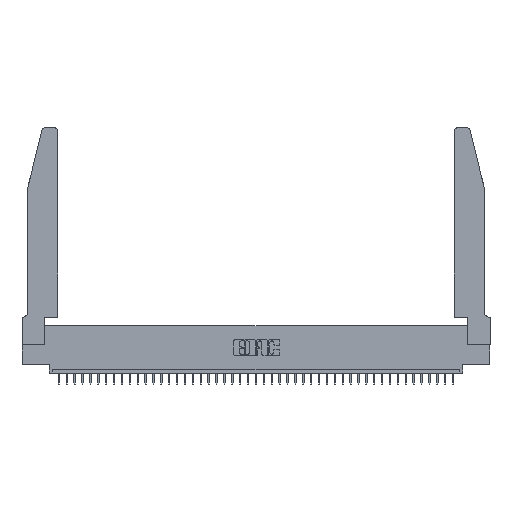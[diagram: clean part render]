
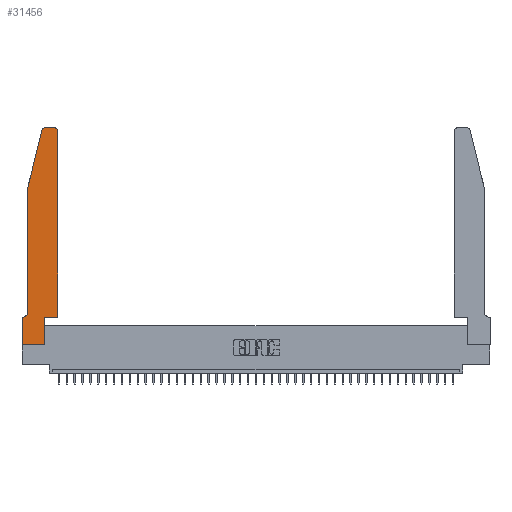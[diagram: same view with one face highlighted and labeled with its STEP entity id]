
A CAD part, top view. The second image highlights one B-rep face of the part: STEP entity #31456.
In plain terms, the highlighted planar face has unit normal (0, 0, 1).
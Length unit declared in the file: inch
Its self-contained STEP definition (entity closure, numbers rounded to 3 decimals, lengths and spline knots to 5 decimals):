
#606 = ORIENTED_EDGE ( 'NONE', *, *, #36842, .T. ) ;
#1045 = LINE ( 'NONE', #23851, #20287 ) ;
#1211 = ORIENTED_EDGE ( 'NONE', *, *, #30237, .T. ) ;
#1244 = CARTESIAN_POINT ( 'NONE',  ( 0.4505, 2.72, 0.37 ) ) ;
#2328 = LINE ( 'NONE', #15305, #37994 ) ;
#2401 = DIRECTION ( 'NONE',  ( 1., 0., 0. ) ) ;
#3042 = CARTESIAN_POINT ( 'NONE',  ( 0.0755, 2., 0.37 ) ) ;
#3442 = VERTEX_POINT ( 'NONE', #22814 ) ;
#3602 = VERTEX_POINT ( 'NONE', #1244 ) ;
#4045 = ORIENTED_EDGE ( 'NONE', *, *, #16039, .T. ) ;
#4070 = VECTOR ( 'NONE', #5723, 39.37008 ) ;
#4198 = ORIENTED_EDGE ( 'NONE', *, *, #23228, .T. ) ;
#4485 = VERTEX_POINT ( 'NONE', #30948 ) ;
#4670 = PLANE ( 'NONE',  #37816 ) ;
#5023 = ORIENTED_EDGE ( 'NONE', *, *, #5055, .T. ) ;
#5055 = EDGE_CURVE ( 'NONE', #14122, #22000, #2328, .T. ) ;
#5507 = EDGE_CURVE ( 'NONE', #41959, #19630, #41713, .T. ) ;
#5723 = DIRECTION ( 'NONE',  ( -1., 0., 0. ) ) ;
#5950 = EDGE_CURVE ( 'NONE', #22000, #36508, #8387, .T. ) ;
#6089 = CARTESIAN_POINT ( 'NONE',  ( 0.0755, 0.42, 0.37 ) ) ;
#6306 = CARTESIAN_POINT ( 'NONE',  ( 0.4205, 2.75, 0.37 ) ) ;
#6488 = EDGE_CURVE ( 'NONE', #36508, #39831, #25980, .T. ) ;
#6580 = DIRECTION ( 'NONE',  ( 1., 0., 0. ) ) ;
#6713 = VERTEX_POINT ( 'NONE', #30853 ) ;
#7894 = CARTESIAN_POINT ( 'NONE',  ( 0.4505, 0.35, 0.37 ) ) ;
#8236 = CARTESIAN_POINT ( 'NONE',  ( 0.0755, 0.35, 0.37 ) ) ;
#8387 = LINE ( 'NONE', #15000, #8738 ) ;
#8738 = VECTOR ( 'NONE', #38462, 39.37008 ) ;
#9120 = DIRECTION ( 'NONE',  ( 1., 0., 0. ) ) ;
#9305 = ORIENTED_EDGE ( 'NONE', *, *, #5507, .T. ) ;
#10061 = CARTESIAN_POINT ( 'NONE',  ( 0.0055, 0.42, 0.37 ) ) ;
#10127 = ORIENTED_EDGE ( 'NONE', *, *, #6488, .T. ) ;
#12064 = CARTESIAN_POINT ( 'NONE',  ( 0.2865, 0., 0.37 ) ) ;
#12339 = ORIENTED_EDGE ( 'NONE', *, *, #30399, .T. ) ;
#12459 = DIRECTION ( 'NONE',  ( 0., -1., 0. ) ) ;
#13036 = EDGE_CURVE ( 'NONE', #6713, #21126, #40873, .T. ) ;
#13082 = CARTESIAN_POINT ( 'NONE',  ( 0.0755, 2., 0.37 ) ) ;
#13480 = ORIENTED_EDGE ( 'NONE', *, *, #25115, .T. ) ;
#14122 = VERTEX_POINT ( 'NONE', #41504 ) ;
#15000 = CARTESIAN_POINT ( 'NONE',  ( 0.2865, 0.35, 0.37 ) ) ;
#15305 = CARTESIAN_POINT ( 'NONE',  ( 0., 0., 0.37 ) ) ;
#16039 = EDGE_CURVE ( 'NONE', #39831, #3602, #30928, .T. ) ;
#17051 = DIRECTION ( 'NONE',  ( 0., -1., 0. ) ) ;
#17083 = DIRECTION ( 'NONE',  ( -1., 0., 0. ) ) ;
#17135 = AXIS2_PLACEMENT_3D ( 'NONE', #31390, #18594, #2401 ) ;
#18223 = CARTESIAN_POINT ( 'NONE',  ( 0., 0.35, 0.37 ) ) ;
#18594 = DIRECTION ( 'NONE',  ( 0., 0., 1. ) ) ;
#18669 = DIRECTION ( 'NONE',  ( 1., 0., 0. ) ) ;
#19284 = VECTOR ( 'NONE', #28273, 39.37008 ) ;
#19527 = DIRECTION ( 'NONE',  ( 0., 0., 1. ) ) ;
#19536 = DIRECTION ( 'NONE',  ( 1., 0., 0. ) ) ;
#19630 = VERTEX_POINT ( 'NONE', #6089 ) ;
#19862 = CARTESIAN_POINT ( 'NONE',  ( 0.2865, 0.35, 0.37 ) ) ;
#20282 = DIRECTION ( 'NONE',  ( 0., 0., -1. ) ) ;
#20287 = VECTOR ( 'NONE', #17051, 39.37008 ) ;
#20351 = VECTOR ( 'NONE', #6580, 39.37008 ) ;
#20689 = CIRCLE ( 'NONE', #39810, 0.07 ) ;
#21126 = VERTEX_POINT ( 'NONE', #18223 ) ;
#22000 = VERTEX_POINT ( 'NONE', #12064 ) ;
#22293 = DIRECTION ( 'NONE',  ( 0., 0., 1. ) ) ;
#22575 = CARTESIAN_POINT ( 'NONE',  ( 0.2605, 2.75, 0.37 ) ) ;
#22684 = VECTOR ( 'NONE', #40524, 39.37008 ) ;
#22814 = CARTESIAN_POINT ( 'NONE',  ( 0.25487, 2.72718, 0.37 ) ) ;
#22994 = CARTESIAN_POINT ( 'NONE',  ( 0.4505, 0.35, 0.37 ) ) ;
#23228 = EDGE_CURVE ( 'NONE', #21126, #14122, #1045, .T. ) ;
#23851 = CARTESIAN_POINT ( 'NONE',  ( 0., 0., 0.37 ) ) ;
#24063 = CARTESIAN_POINT ( 'NONE',  ( 0., 0.35, 0.37 ) ) ;
#25115 = EDGE_CURVE ( 'NONE', #3602, #39300, #33986, .T. ) ;
#25980 = LINE ( 'NONE', #22994, #20351 ) ;
#27357 = CIRCLE ( 'NONE', #17135, 0.03 ) ;
#27394 = ORIENTED_EDGE ( 'NONE', *, *, #13036, .T. ) ;
#27670 = EDGE_LOOP ( 'NONE', ( #606, #28945, #1211, #9305, #12339, #27394, #4198, #5023, #42101, #10127, #4045, #13480 ) ) ;
#28273 = DIRECTION ( 'NONE',  ( -1., 0., 0. ) ) ;
#28945 = ORIENTED_EDGE ( 'NONE', *, *, #41158, .T. ) ;
#30237 = EDGE_CURVE ( 'NONE', #3442, #41959, #38646, .T. ) ;
#30399 = EDGE_CURVE ( 'NONE', #19630, #6713, #20689, .T. ) ;
#30853 = CARTESIAN_POINT ( 'NONE',  ( 0.0055, 0.35, 0.37 ) ) ;
#30928 = LINE ( 'NONE', #7894, #22684 ) ;
#30948 = CARTESIAN_POINT ( 'NONE',  ( 0.284, 2.75, 0.37 ) ) ;
#31390 = CARTESIAN_POINT ( 'NONE',  ( 0.284, 2.72, 0.37 ) ) ;
#31456 = ADVANCED_FACE ( 'NONE', ( #40291 ), #4670, .T. ) ;
#31618 = DIRECTION ( 'NONE',  ( -0.239, -0.971, 0. ) ) ;
#33986 = CIRCLE ( 'NONE', #37390, 0.03 ) ;
#34327 = VECTOR ( 'NONE', #31618, 39.37008 ) ;
#36508 = VERTEX_POINT ( 'NONE', #19862 ) ;
#36650 = VECTOR ( 'NONE', #12459, 39.37008 ) ;
#36725 = CARTESIAN_POINT ( 'NONE',  ( 0.4505, 0.35, 0.37 ) ) ;
#36842 = EDGE_CURVE ( 'NONE', #39300, #4485, #41974, .T. ) ;
#37390 = AXIS2_PLACEMENT_3D ( 'NONE', #41924, #22293, #19536 ) ;
#37816 = AXIS2_PLACEMENT_3D ( 'NONE', #24063, #19527, #18669 ) ;
#37994 = VECTOR ( 'NONE', #9120, 39.37008 ) ;
#38462 = DIRECTION ( 'NONE',  ( 0., 1., 0. ) ) ;
#38512 = CARTESIAN_POINT ( 'NONE',  ( 0.0755, 2., 0.37 ) ) ;
#38646 = LINE ( 'NONE', #3042, #34327 ) ;
#39300 = VERTEX_POINT ( 'NONE', #6306 ) ;
#39810 = AXIS2_PLACEMENT_3D ( 'NONE', #10061, #20282, #17083 ) ;
#39831 = VERTEX_POINT ( 'NONE', #36725 ) ;
#40291 = FACE_OUTER_BOUND ( 'NONE', #27670, .T. ) ;
#40524 = DIRECTION ( 'NONE',  ( 0., 1., 0. ) ) ;
#40873 = LINE ( 'NONE', #8236, #19284 ) ;
#41158 = EDGE_CURVE ( 'NONE', #4485, #3442, #27357, .T. ) ;
#41504 = CARTESIAN_POINT ( 'NONE',  ( 0., 0., 0.37 ) ) ;
#41713 = LINE ( 'NONE', #38512, #36650 ) ;
#41924 = CARTESIAN_POINT ( 'NONE',  ( 0.4205, 2.72, 0.37 ) ) ;
#41959 = VERTEX_POINT ( 'NONE', #13082 ) ;
#41974 = LINE ( 'NONE', #22575, #4070 ) ;
#42101 = ORIENTED_EDGE ( 'NONE', *, *, #5950, .T. ) ;
